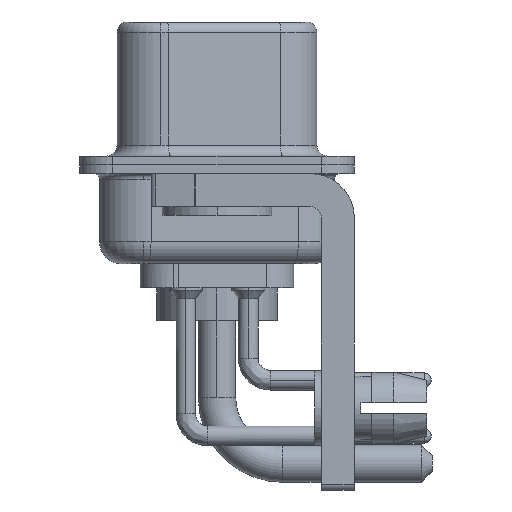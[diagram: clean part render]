
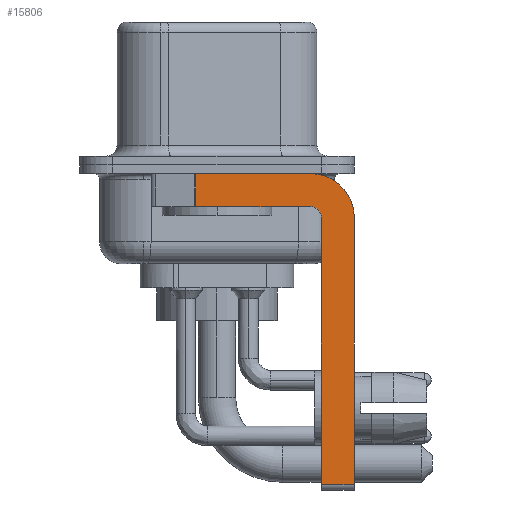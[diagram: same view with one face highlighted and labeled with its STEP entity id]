
A CAD part, left-side view. The second image highlights one B-rep face of the part: STEP entity #15806.
In plain terms, the highlighted planar face has unit normal (-1, 0, 0).
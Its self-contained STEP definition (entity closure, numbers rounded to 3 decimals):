
#438 = CIRCLE ( 'NONE', #5364, 0.5 ) ;
#702 = DIRECTION ( 'NONE',  ( 1., 0., 0. ) ) ;
#704 = VECTOR ( 'NONE', #5483, 1000. ) ;
#909 = EDGE_CURVE ( 'NONE', #8146, #1725, #19171, .T. ) ;
#1606 = LINE ( 'NONE', #6757, #19812 ) ;
#1706 = LINE ( 'NONE', #8187, #10294 ) ;
#1725 = VERTEX_POINT ( 'NONE', #8480 ) ;
#1876 = LINE ( 'NONE', #13209, #14468 ) ;
#1941 = EDGE_CURVE ( 'NONE', #9180, #15124, #438, .T. ) ;
#2100 = CARTESIAN_POINT ( 'NONE',  ( -2.9, -4.25, -0.4 ) ) ;
#2257 = ORIENTED_EDGE ( 'NONE', *, *, #16551, .T. ) ;
#2271 = CARTESIAN_POINT ( 'NONE',  ( -2.9, -4.75, -2.4 ) ) ;
#3598 = PLANE ( 'NONE',  #13381 ) ;
#3672 = EDGE_CURVE ( 'NONE', #13151, #8146, #7123, .T. ) ;
#4164 = EDGE_LOOP ( 'NONE', ( #17409, #2257, #16688, #7446, #12079, #12629, #6793, #10774 ) ) ;
#4798 = VECTOR ( 'NONE', #16860, 1000. ) ;
#4999 = CARTESIAN_POINT ( 'NONE',  ( -2.9, -4.75, -14.8 ) ) ;
#5353 = DIRECTION ( 'NONE',  ( 1., 0., 0. ) ) ;
#5364 = AXIS2_PLACEMENT_3D ( 'NONE', #18910, #15501, #5507 ) ;
#5483 = DIRECTION ( 'NONE',  ( 0., -1., 0. ) ) ;
#5507 = DIRECTION ( 'NONE',  ( 0., 0., 1. ) ) ;
#5662 = DIRECTION ( 'NONE',  ( 0., 0., -1. ) ) ;
#6536 = DIRECTION ( 'NONE',  ( 0., 1., 0. ) ) ;
#6593 = DIRECTION ( 'NONE',  ( 0., 0., -1. ) ) ;
#6757 = CARTESIAN_POINT ( 'NONE',  ( -2.9, -6.25, -2.4 ) ) ;
#6793 = ORIENTED_EDGE ( 'NONE', *, *, #21066, .F. ) ;
#7064 = CARTESIAN_POINT ( 'NONE',  ( -2.9, 0.978, -0.4 ) ) ;
#7123 = LINE ( 'NONE', #10432, #704 ) ;
#7132 = VECTOR ( 'NONE', #8745, 1000. ) ;
#7446 = ORIENTED_EDGE ( 'NONE', *, *, #1941, .F. ) ;
#7599 = CARTESIAN_POINT ( 'NONE',  ( -2.9, -4.25, -1.9 ) ) ;
#7765 = EDGE_CURVE ( 'NONE', #15124, #9227, #1706, .T. ) ;
#8146 = VERTEX_POINT ( 'NONE', #2100 ) ;
#8187 = CARTESIAN_POINT ( 'NONE',  ( -2.9, -4.25, -1.9 ) ) ;
#8480 = CARTESIAN_POINT ( 'NONE',  ( -2.9, -6.25, -2.4 ) ) ;
#8745 = DIRECTION ( 'NONE',  ( 0., 0., 1. ) ) ;
#9180 = VERTEX_POINT ( 'NONE', #2271 ) ;
#9227 = VERTEX_POINT ( 'NONE', #19528 ) ;
#10068 = LINE ( 'NONE', #4999, #7132 ) ;
#10163 = CARTESIAN_POINT ( 'NONE',  ( -2.9, -4.25, -14.55 ) ) ;
#10294 = VECTOR ( 'NONE', #6536, 1000. ) ;
#10376 = LINE ( 'NONE', #10163, #4798 ) ;
#10432 = CARTESIAN_POINT ( 'NONE',  ( -2.9, 3., -0.4 ) ) ;
#10515 = FACE_OUTER_BOUND ( 'NONE', #4164, .T. ) ;
#10722 = CARTESIAN_POINT ( 'NONE',  ( -2.9, -4.75, -14.55 ) ) ;
#10774 = ORIENTED_EDGE ( 'NONE', *, *, #909, .F. ) ;
#12067 = DIRECTION ( 'NONE',  ( 0., 0., -1. ) ) ;
#12079 = ORIENTED_EDGE ( 'NONE', *, *, #19567, .F. ) ;
#12629 = ORIENTED_EDGE ( 'NONE', *, *, #13091, .T. ) ;
#13053 = DIRECTION ( 'NONE',  ( 0., 0., -1. ) ) ;
#13091 = EDGE_CURVE ( 'NONE', #17568, #14294, #10376, .T. ) ;
#13151 = VERTEX_POINT ( 'NONE', #7064 ) ;
#13209 = CARTESIAN_POINT ( 'NONE',  ( -2.9, 0.978, -1.9 ) ) ;
#13381 = AXIS2_PLACEMENT_3D ( 'NONE', #20403, #5353, #12067 ) ;
#14294 = VERTEX_POINT ( 'NONE', #14707 ) ;
#14468 = VECTOR ( 'NONE', #6593, 1000. ) ;
#14707 = CARTESIAN_POINT ( 'NONE',  ( -2.9, -6.25, -14.55 ) ) ;
#15124 = VERTEX_POINT ( 'NONE', #7599 ) ;
#15501 = DIRECTION ( 'NONE',  ( -1., 0., 0. ) ) ;
#15557 = CARTESIAN_POINT ( 'NONE',  ( -2.9, -4.25, -2.4 ) ) ;
#15806 = ADVANCED_FACE ( 'NONE', ( #10515 ), #3598, .F. ) ;
#16551 = EDGE_CURVE ( 'NONE', #13151, #9227, #1876, .T. ) ;
#16688 = ORIENTED_EDGE ( 'NONE', *, *, #7765, .F. ) ;
#16860 = DIRECTION ( 'NONE',  ( 0., -1., 0. ) ) ;
#17409 = ORIENTED_EDGE ( 'NONE', *, *, #3672, .F. ) ;
#17568 = VERTEX_POINT ( 'NONE', #10722 ) ;
#18910 = CARTESIAN_POINT ( 'NONE',  ( -2.9, -4.25, -2.4 ) ) ;
#19171 = CIRCLE ( 'NONE', #20573, 2. ) ;
#19528 = CARTESIAN_POINT ( 'NONE',  ( -2.9, 0.978, -1.9 ) ) ;
#19567 = EDGE_CURVE ( 'NONE', #17568, #9180, #10068, .T. ) ;
#19812 = VECTOR ( 'NONE', #13053, 1000. ) ;
#20403 = CARTESIAN_POINT ( 'NONE',  ( -2.9, -4.25, -2.4 ) ) ;
#20573 = AXIS2_PLACEMENT_3D ( 'NONE', #15557, #702, #5662 ) ;
#21066 = EDGE_CURVE ( 'NONE', #1725, #14294, #1606, .T. ) ;
